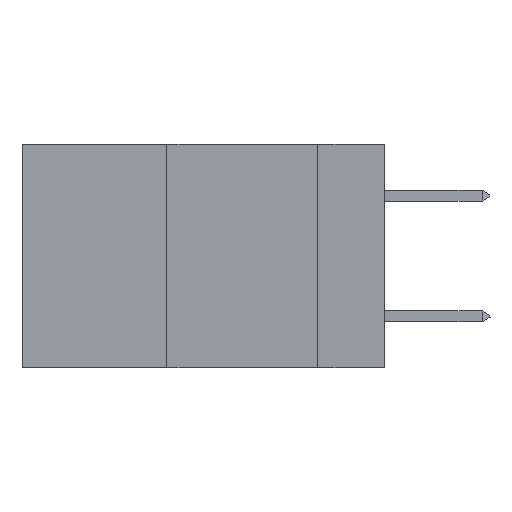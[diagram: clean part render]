
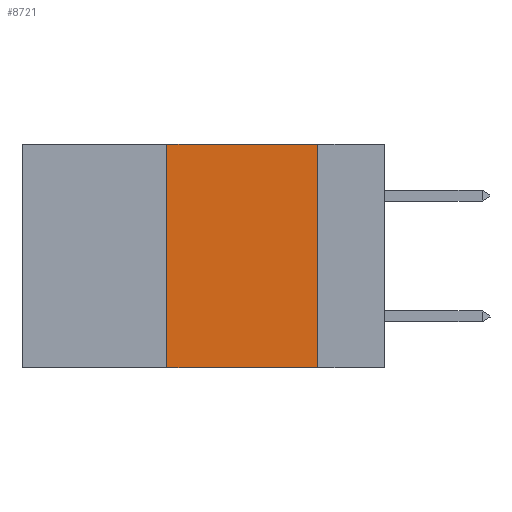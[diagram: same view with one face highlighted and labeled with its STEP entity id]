
A CAD part, left-side view. The second image highlights one B-rep face of the part: STEP entity #8721.
In plain terms, the highlighted planar face has unit normal (-1, 0, 0).
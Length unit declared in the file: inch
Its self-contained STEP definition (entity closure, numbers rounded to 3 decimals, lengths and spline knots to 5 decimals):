
#937 = EDGE_CURVE ( 'NONE', #2322, #7394, #14435, .T. ) ;
#990 = CARTESIAN_POINT ( 'NONE',  ( 0., 0.6, 0. ) ) ;
#1389 = LINE ( 'NONE', #990, #17979 ) ;
#1657 = VERTEX_POINT ( 'NONE', #7152 ) ;
#2322 = VERTEX_POINT ( 'NONE', #20049 ) ;
#2919 = CARTESIAN_POINT ( 'NONE',  ( 0., 0.6, -0.37 ) ) ;
#3657 = ORIENTED_EDGE ( 'NONE', *, *, #937, .F. ) ;
#4993 = CARTESIAN_POINT ( 'NONE',  ( 0., 0.36, 0. ) ) ;
#5972 = VECTOR ( 'NONE', #19325, 39.37008 ) ;
#6237 = PLANE ( 'NONE',  #15892 ) ;
#6760 = EDGE_CURVE ( 'NONE', #2322, #1657, #8257, .T. ) ;
#7001 = EDGE_CURVE ( 'NONE', #7394, #14606, #1389, .T. ) ;
#7152 = CARTESIAN_POINT ( 'NONE',  ( 0., 0.11, -0.37 ) ) ;
#7394 = VERTEX_POINT ( 'NONE', #4993 ) ;
#8090 = EDGE_LOOP ( 'NONE', ( #11233, #15344, #3657, #12046 ) ) ;
#8257 = LINE ( 'NONE', #2919, #16278 ) ;
#8721 = ADVANCED_FACE ( 'NONE', ( #15482 ), #6237, .F. ) ;
#9289 = DIRECTION ( 'NONE',  ( 0., -1., 0. ) ) ;
#9454 = DIRECTION ( 'NONE',  ( 1., 0., 0. ) ) ;
#10245 = LINE ( 'NONE', #16214, #5972 ) ;
#10391 = VECTOR ( 'NONE', #18964, 39.37008 ) ;
#11233 = ORIENTED_EDGE ( 'NONE', *, *, #19985, .F. ) ;
#11784 = CARTESIAN_POINT ( 'NONE',  ( 0., 0.11, 0. ) ) ;
#12046 = ORIENTED_EDGE ( 'NONE', *, *, #6760, .T. ) ;
#14435 = LINE ( 'NONE', #15720, #10391 ) ;
#14606 = VERTEX_POINT ( 'NONE', #11784 ) ;
#15344 = ORIENTED_EDGE ( 'NONE', *, *, #7001, .F. ) ;
#15482 = FACE_OUTER_BOUND ( 'NONE', #8090, .T. ) ;
#15720 = CARTESIAN_POINT ( 'NONE',  ( 0., 0.36, 0. ) ) ;
#15892 = AXIS2_PLACEMENT_3D ( 'NONE', #17307, #9454, #20498 ) ;
#16214 = CARTESIAN_POINT ( 'NONE',  ( 0., 0.11, 0. ) ) ;
#16278 = VECTOR ( 'NONE', #9289, 39.37008 ) ;
#17307 = CARTESIAN_POINT ( 'NONE',  ( 0., 0.6, 0. ) ) ;
#17979 = VECTOR ( 'NONE', #18737, 39.37008 ) ;
#18737 = DIRECTION ( 'NONE',  ( 0., -1., 0. ) ) ;
#18964 = DIRECTION ( 'NONE',  ( 0., 0., 1. ) ) ;
#19325 = DIRECTION ( 'NONE',  ( 0., 0., -1. ) ) ;
#19985 = EDGE_CURVE ( 'NONE', #14606, #1657, #10245, .T. ) ;
#20049 = CARTESIAN_POINT ( 'NONE',  ( 0., 0.36, -0.37 ) ) ;
#20498 = DIRECTION ( 'NONE',  ( 0., 0., -1. ) ) ;
